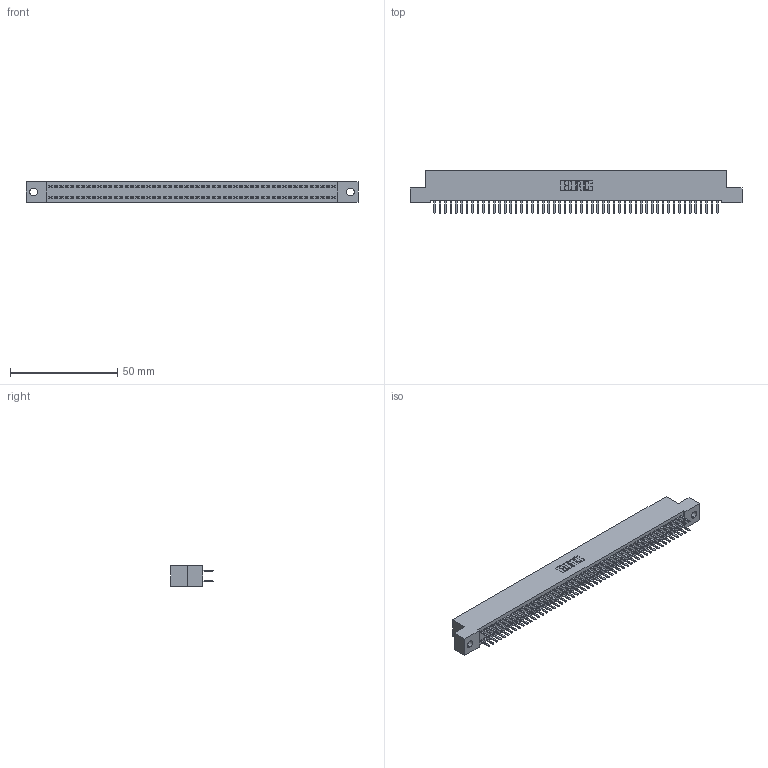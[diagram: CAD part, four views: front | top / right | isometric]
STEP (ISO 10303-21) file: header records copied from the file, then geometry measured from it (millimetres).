
FILE_DESCRIPTION (( 'STEP AP203' ), '1' );
FILE_NAME ('342-106-520-202.STEP', '2019-10-04T19:02:30', ( '' ), ( '' ), 'SwSTEP 2.0', 'SolidWorks 2016', '' );
FILE_SCHEMA (( 'CONFIG_CONTROL_DESIGN' ));
Length unit declared in the file: inch
Products named in the file (3): 342 Part_.128 Slot; 345-292-001_345-293-120; 342-106-520-202
Assembly tree (107 placements, depth 2):
  342-106-520-202
    342 Part_.128 Slot
    345-292-001_345-293-120  x106
Bounding box: 154.94 x 20.02 x 9.4 mm (x, y, z)
Volume: 13874.7 mm3; surface area: 22505.1 mm2
Topology: 107 solids, 107 shells, 6050 faces, 17589 edges, 11442 vertices
Faces by surface type: plane 4098, cylinder 1952
Entity records: 32791 total; most frequent: CARTESIAN_POINT 5434, ORIENTED_EDGE 5358, DIRECTION 4611, EDGE_CURVE 2679, LINE 2547, VECTOR 2547, VERTEX_POINT 1782, AXIS2_PLACEMENT_3D 1032
